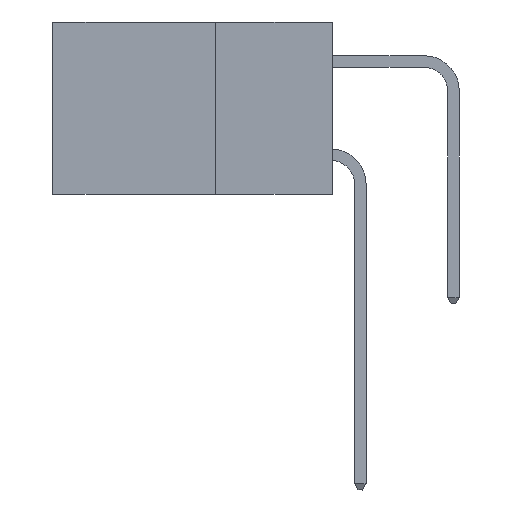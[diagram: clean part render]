
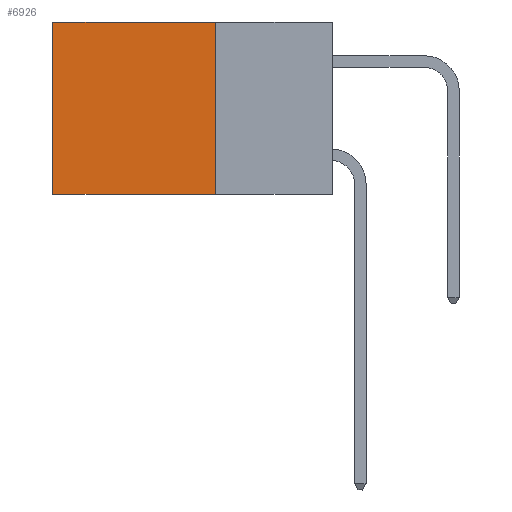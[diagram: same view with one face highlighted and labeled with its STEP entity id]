
A CAD part, left-side view. The second image highlights one B-rep face of the part: STEP entity #6926.
In plain terms, the highlighted planar face has unit normal (-1, 0, 0).
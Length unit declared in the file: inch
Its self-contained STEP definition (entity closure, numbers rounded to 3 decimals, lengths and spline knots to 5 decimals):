
#359 = VERTEX_POINT ( 'NONE', #7334 ) ;
#606 = EDGE_CURVE ( 'NONE', #27768, #20710, #1344, .T. ) ;
#1344 = LINE ( 'NONE', #13024, #3110 ) ;
#2144 = EDGE_LOOP ( 'NONE', ( #23677, #8192, #25708, #4846 ) ) ;
#2231 = CARTESIAN_POINT ( 'NONE',  ( 0.2615, 0.25, 0. ) ) ;
#2926 = LINE ( 'NONE', #26867, #13218 ) ;
#3067 = VECTOR ( 'NONE', #20026, 39.37008 ) ;
#3110 = VECTOR ( 'NONE', #8057, 39.37008 ) ;
#4846 = ORIENTED_EDGE ( 'NONE', *, *, #26467, .T. ) ;
#5659 = LINE ( 'NONE', #5953, #24576 ) ;
#5953 = CARTESIAN_POINT ( 'NONE',  ( 0.2615, 0.25, -0.37 ) ) ;
#6926 = ADVANCED_FACE ( 'NONE', ( #13583 ), #22451, .F. ) ;
#6999 = DIRECTION ( 'NONE',  ( 0., 0., -1. ) ) ;
#7334 = CARTESIAN_POINT ( 'NONE',  ( 0.2615, 0.6, 0. ) ) ;
#8057 = DIRECTION ( 'NONE',  ( 0., 1., 0. ) ) ;
#8192 = ORIENTED_EDGE ( 'NONE', *, *, #606, .F. ) ;
#9114 = VERTEX_POINT ( 'NONE', #12207 ) ;
#10714 = CARTESIAN_POINT ( 'NONE',  ( 0.2615, 0.6, -0.37 ) ) ;
#12207 = CARTESIAN_POINT ( 'NONE',  ( 0.2615, 0.25, 0. ) ) ;
#13024 = CARTESIAN_POINT ( 'NONE',  ( 0.2615, 0.25, -0.37 ) ) ;
#13218 = VECTOR ( 'NONE', #20291, 39.37008 ) ;
#13583 = FACE_OUTER_BOUND ( 'NONE', #2144, .T. ) ;
#14909 = EDGE_CURVE ( 'NONE', #9114, #27768, #5659, .T. ) ;
#17934 = CARTESIAN_POINT ( 'NONE',  ( 0.2615, 0.25, -0.37 ) ) ;
#20026 = DIRECTION ( 'NONE',  ( 0., 1., 0. ) ) ;
#20269 = DIRECTION ( 'NONE',  ( 1., 0., 0. ) ) ;
#20291 = DIRECTION ( 'NONE',  ( 0., 0., -1. ) ) ;
#20710 = VERTEX_POINT ( 'NONE', #10714 ) ;
#21503 = AXIS2_PLACEMENT_3D ( 'NONE', #17934, #20269, #6999 ) ;
#22451 = PLANE ( 'NONE',  #21503 ) ;
#23677 = ORIENTED_EDGE ( 'NONE', *, *, #24230, .T. ) ;
#24230 = EDGE_CURVE ( 'NONE', #359, #20710, #2926, .T. ) ;
#24444 = CARTESIAN_POINT ( 'NONE',  ( 0.2615, 0.25, -0.37 ) ) ;
#24576 = VECTOR ( 'NONE', #26093, 39.37008 ) ;
#24836 = LINE ( 'NONE', #2231, #3067 ) ;
#25708 = ORIENTED_EDGE ( 'NONE', *, *, #14909, .F. ) ;
#26093 = DIRECTION ( 'NONE',  ( 0., 0., -1. ) ) ;
#26467 = EDGE_CURVE ( 'NONE', #9114, #359, #24836, .T. ) ;
#26867 = CARTESIAN_POINT ( 'NONE',  ( 0.2615, 0.6, -0.37 ) ) ;
#27768 = VERTEX_POINT ( 'NONE', #24444 ) ;
